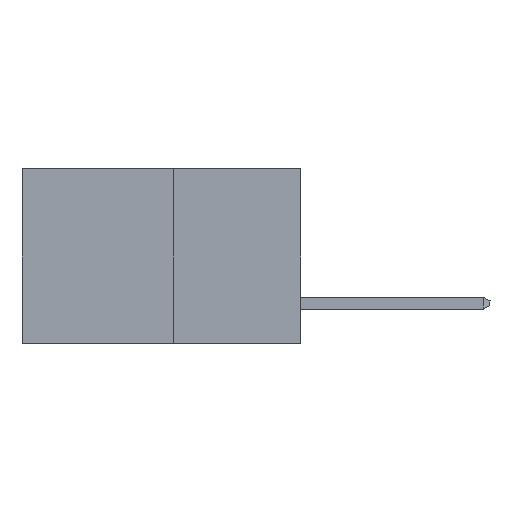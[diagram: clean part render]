
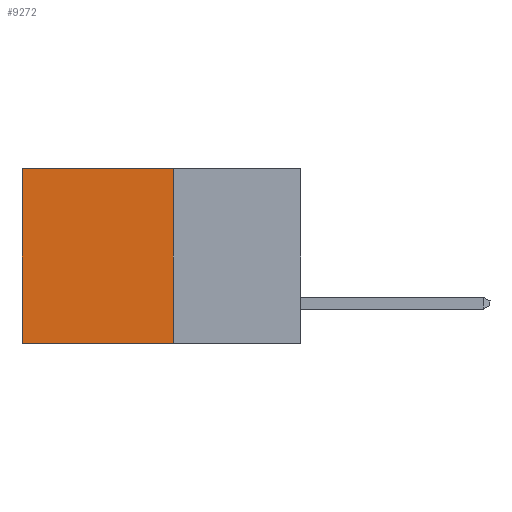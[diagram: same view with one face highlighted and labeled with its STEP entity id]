
A CAD part, left-side view. The second image highlights one B-rep face of the part: STEP entity #9272.
In plain terms, the highlighted planar face has unit normal (-1, 0, 0).
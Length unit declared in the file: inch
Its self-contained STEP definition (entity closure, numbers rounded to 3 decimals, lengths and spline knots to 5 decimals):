
#645 = DIRECTION ( 'NONE',  ( 1., 0., 0. ) ) ;
#1551 = DIRECTION ( 'NONE',  ( 0., 0., -1. ) ) ;
#1568 = CARTESIAN_POINT ( 'NONE',  ( 0.277, 0.59, -0.37 ) ) ;
#1601 = AXIS2_PLACEMENT_3D ( 'NONE', #9840, #645, #7853 ) ;
#2151 = EDGE_LOOP ( 'NONE', ( #9193, #2258, #8090, #8732 ) ) ;
#2258 = ORIENTED_EDGE ( 'NONE', *, *, #6612, .F. ) ;
#2505 = CARTESIAN_POINT ( 'NONE',  ( 0.277, 0.59, -0.37 ) ) ;
#3772 = DIRECTION ( 'NONE',  ( 0., 0., -1. ) ) ;
#4494 = EDGE_CURVE ( 'NONE', #8766, #5458, #9743, .T. ) ;
#5458 = VERTEX_POINT ( 'NONE', #2505 ) ;
#6612 = EDGE_CURVE ( 'NONE', #7369, #5458, #7482, .T. ) ;
#6683 = DIRECTION ( 'NONE',  ( 0., 1., 0. ) ) ;
#6802 = DIRECTION ( 'NONE',  ( 0., 1., 0. ) ) ;
#6887 = CARTESIAN_POINT ( 'NONE',  ( 0.277, 0.27, -0.37 ) ) ;
#6891 = CARTESIAN_POINT ( 'NONE',  ( 0.277, 0.27, -0.37 ) ) ;
#7369 = VERTEX_POINT ( 'NONE', #6887 ) ;
#7471 = LINE ( 'NONE', #12704, #9842 ) ;
#7482 = LINE ( 'NONE', #6891, #12202 ) ;
#7708 = VERTEX_POINT ( 'NONE', #12395 ) ;
#7853 = DIRECTION ( 'NONE',  ( 0., 0., -1. ) ) ;
#8090 = ORIENTED_EDGE ( 'NONE', *, *, #12259, .F. ) ;
#8212 = VECTOR ( 'NONE', #3772, 39.37008 ) ;
#8732 = ORIENTED_EDGE ( 'NONE', *, *, #10907, .T. ) ;
#8766 = VERTEX_POINT ( 'NONE', #10882 ) ;
#8849 = CARTESIAN_POINT ( 'NONE',  ( 0.277, 0.27, -0.37 ) ) ;
#9042 = FACE_OUTER_BOUND ( 'NONE', #2151, .T. ) ;
#9193 = ORIENTED_EDGE ( 'NONE', *, *, #4494, .T. ) ;
#9272 = ADVANCED_FACE ( 'NONE', ( #9042 ), #9790, .F. ) ;
#9743 = LINE ( 'NONE', #1568, #12111 ) ;
#9790 = PLANE ( 'NONE',  #1601 ) ;
#9840 = CARTESIAN_POINT ( 'NONE',  ( 0.277, 0.27, -0.37 ) ) ;
#9842 = VECTOR ( 'NONE', #6683, 39.37008 ) ;
#10882 = CARTESIAN_POINT ( 'NONE',  ( 0.277, 0.59, 0. ) ) ;
#10907 = EDGE_CURVE ( 'NONE', #7708, #8766, #7471, .T. ) ;
#10912 = LINE ( 'NONE', #8849, #8212 ) ;
#12111 = VECTOR ( 'NONE', #1551, 39.37008 ) ;
#12202 = VECTOR ( 'NONE', #6802, 39.37008 ) ;
#12259 = EDGE_CURVE ( 'NONE', #7708, #7369, #10912, .T. ) ;
#12395 = CARTESIAN_POINT ( 'NONE',  ( 0.277, 0.27, 0. ) ) ;
#12704 = CARTESIAN_POINT ( 'NONE',  ( 0.277, 0.27, 0. ) ) ;
